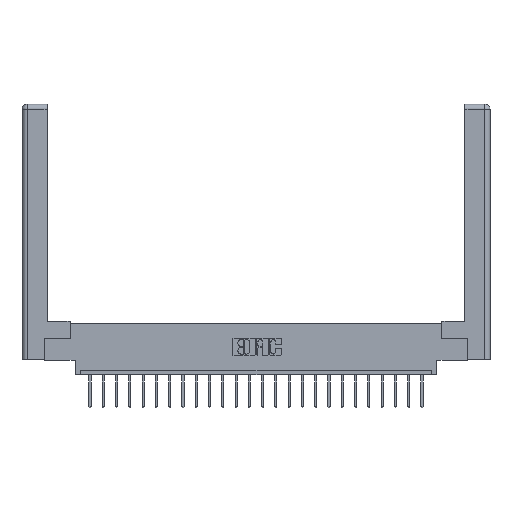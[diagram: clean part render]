
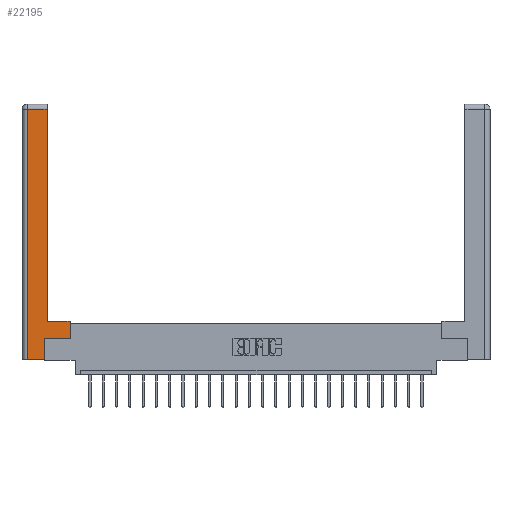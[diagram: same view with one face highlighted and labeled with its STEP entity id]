
A CAD part, top view. The second image highlights one B-rep face of the part: STEP entity #22195.
In plain terms, the highlighted planar face has unit normal (0, 0, 1).
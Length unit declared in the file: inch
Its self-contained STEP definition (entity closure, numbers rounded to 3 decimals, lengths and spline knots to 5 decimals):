
#1099 = ORIENTED_EDGE ( 'NONE', *, *, #1779, .T. ) ;
#1216 = PLANE ( 'NONE',  #20299 ) ;
#1779 = EDGE_CURVE ( 'NONE', #22459, #20631, #23409, .T. ) ;
#1830 = EDGE_CURVE ( 'NONE', #4709, #16460, #19902, .T. ) ;
#2073 = CARTESIAN_POINT ( 'NONE',  ( 0.565, 0.45, 0. ) ) ;
#2435 = EDGE_CURVE ( 'NONE', #20631, #13533, #8221, .T. ) ;
#2973 = CARTESIAN_POINT ( 'NONE',  ( 0.295, 0.45, 0. ) ) ;
#3324 = CARTESIAN_POINT ( 'NONE',  ( 0.265, 0.245, 0. ) ) ;
#3730 = CARTESIAN_POINT ( 'NONE',  ( 0.565, 0.45, 0. ) ) ;
#4175 = CARTESIAN_POINT ( 'NONE',  ( 0.0615, 0., 0. ) ) ;
#4709 = VERTEX_POINT ( 'NONE', #2073 ) ;
#5572 = DIRECTION ( 'NONE',  ( 0., -1., 0. ) ) ;
#6541 = CARTESIAN_POINT ( 'NONE',  ( 0.295, 0.45, 0. ) ) ;
#7053 = CARTESIAN_POINT ( 'NONE',  ( 0.0615, 2.94, 0. ) ) ;
#7107 = EDGE_CURVE ( 'NONE', #16485, #17298, #20426, .T. ) ;
#7419 = ORIENTED_EDGE ( 'NONE', *, *, #2435, .T. ) ;
#7687 = VECTOR ( 'NONE', #5572, 39.37008 ) ;
#8056 = LINE ( 'NONE', #21738, #22917 ) ;
#8215 = VECTOR ( 'NONE', #12228, 39.37008 ) ;
#8221 = LINE ( 'NONE', #3324, #9939 ) ;
#8436 = ORIENTED_EDGE ( 'NONE', *, *, #24151, .T. ) ;
#8542 = CARTESIAN_POINT ( 'NONE',  ( 0., 0., 0. ) ) ;
#8909 = ORIENTED_EDGE ( 'NONE', *, *, #17214, .T. ) ;
#9024 = DIRECTION ( 'NONE',  ( 0., 1., 0. ) ) ;
#9174 = LINE ( 'NONE', #24196, #14733 ) ;
#9658 = EDGE_CURVE ( 'NONE', #12270, #4709, #16528, .T. ) ;
#9939 = VECTOR ( 'NONE', #9024, 39.37008 ) ;
#10217 = EDGE_LOOP ( 'NONE', ( #11021, #23257, #8909, #1099, #7419, #8436, #22601, #21894 ) ) ;
#10599 = CARTESIAN_POINT ( 'NONE',  ( 0.295, 2.94, 0. ) ) ;
#11021 = ORIENTED_EDGE ( 'NONE', *, *, #22261, .T. ) ;
#11445 = CARTESIAN_POINT ( 'NONE',  ( 0.565, 0.245, 0. ) ) ;
#11798 = VECTOR ( 'NONE', #22515, 39.37008 ) ;
#12228 = DIRECTION ( 'NONE',  ( -1., 0., 0. ) ) ;
#12270 = VERTEX_POINT ( 'NONE', #11445 ) ;
#12528 = DIRECTION ( 'NONE',  ( 1., 0., 0. ) ) ;
#13533 = VERTEX_POINT ( 'NONE', #23929 ) ;
#14167 = DIRECTION ( 'NONE',  ( 1., 0., 0. ) ) ;
#14733 = VECTOR ( 'NONE', #16564, 39.37008 ) ;
#15522 = VECTOR ( 'NONE', #14167, 39.37008 ) ;
#15761 = CARTESIAN_POINT ( 'NONE',  ( 0.0615, 2.94, 0. ) ) ;
#16460 = VERTEX_POINT ( 'NONE', #2973 ) ;
#16485 = VERTEX_POINT ( 'NONE', #10599 ) ;
#16528 = LINE ( 'NONE', #3730, #11798 ) ;
#16564 = DIRECTION ( 'NONE',  ( 0., 1., 0. ) ) ;
#16756 = LINE ( 'NONE', #22094, #7687 ) ;
#17214 = EDGE_CURVE ( 'NONE', #17298, #22459, #16756, .T. ) ;
#17298 = VERTEX_POINT ( 'NONE', #15761 ) ;
#17972 = FACE_OUTER_BOUND ( 'NONE', #10217, .T. ) ;
#18070 = CARTESIAN_POINT ( 'NONE',  ( 0.265, 0., 0. ) ) ;
#18422 = DIRECTION ( 'NONE',  ( -1., 0., 0. ) ) ;
#19815 = DIRECTION ( 'NONE',  ( 0., 0., -1. ) ) ;
#19902 = LINE ( 'NONE', #6541, #8215 ) ;
#20299 = AXIS2_PLACEMENT_3D ( 'NONE', #8542, #19815, #24030 ) ;
#20426 = LINE ( 'NONE', #7053, #21266 ) ;
#20631 = VERTEX_POINT ( 'NONE', #18070 ) ;
#21266 = VECTOR ( 'NONE', #18422, 39.37008 ) ;
#21344 = CARTESIAN_POINT ( 'NONE',  ( 0.265, 0., 0. ) ) ;
#21738 = CARTESIAN_POINT ( 'NONE',  ( 0.565, 0.245, 0. ) ) ;
#21894 = ORIENTED_EDGE ( 'NONE', *, *, #1830, .T. ) ;
#22094 = CARTESIAN_POINT ( 'NONE',  ( 0.0615, 0., 0. ) ) ;
#22195 = ADVANCED_FACE ( 'NONE', ( #17972 ), #1216, .F. ) ;
#22261 = EDGE_CURVE ( 'NONE', #16460, #16485, #9174, .T. ) ;
#22459 = VERTEX_POINT ( 'NONE', #4175 ) ;
#22515 = DIRECTION ( 'NONE',  ( 0., 1., 0. ) ) ;
#22601 = ORIENTED_EDGE ( 'NONE', *, *, #9658, .T. ) ;
#22917 = VECTOR ( 'NONE', #12528, 39.37008 ) ;
#23257 = ORIENTED_EDGE ( 'NONE', *, *, #7107, .T. ) ;
#23409 = LINE ( 'NONE', #21344, #15522 ) ;
#23929 = CARTESIAN_POINT ( 'NONE',  ( 0.265, 0.245, 0. ) ) ;
#24030 = DIRECTION ( 'NONE',  ( -1., 0., 0. ) ) ;
#24151 = EDGE_CURVE ( 'NONE', #13533, #12270, #8056, .T. ) ;
#24196 = CARTESIAN_POINT ( 'NONE',  ( 0.295, 3., 0. ) ) ;
